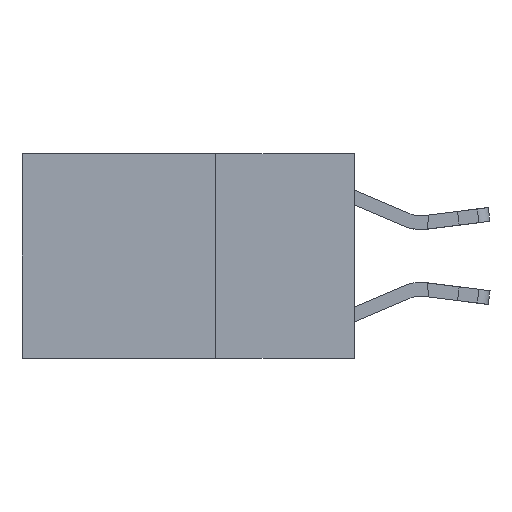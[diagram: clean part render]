
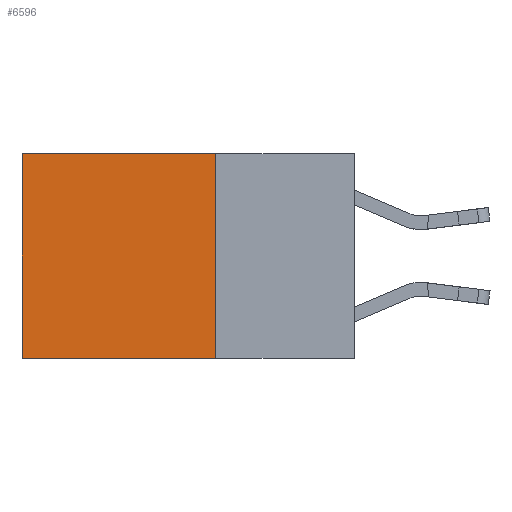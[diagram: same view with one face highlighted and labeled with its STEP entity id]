
A CAD part, left-side view. The second image highlights one B-rep face of the part: STEP entity #6596.
In plain terms, the highlighted planar face has unit normal (-1, 0, 0).
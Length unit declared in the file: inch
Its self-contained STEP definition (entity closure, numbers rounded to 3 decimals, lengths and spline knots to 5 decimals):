
#45 = FACE_OUTER_BOUND ( 'NONE', #14893, .T. ) ;
#304 = ORIENTED_EDGE ( 'NONE', *, *, #19773, .T. ) ;
#1664 = EDGE_CURVE ( 'NONE', #19805, #15341, #19872, .T. ) ;
#1724 = CARTESIAN_POINT ( 'NONE',  ( 0.2625, 0.25, 0. ) ) ;
#1777 = CARTESIAN_POINT ( 'NONE',  ( 0.2625, 0.25, -0.37 ) ) ;
#2190 = VECTOR ( 'NONE', #11734, 39.37008 ) ;
#2728 = LINE ( 'NONE', #18237, #15926 ) ;
#4060 = CARTESIAN_POINT ( 'NONE',  ( 0.2625, 0.6, -0.37 ) ) ;
#5270 = CARTESIAN_POINT ( 'NONE',  ( 0.2625, 0.25, -0.37 ) ) ;
#6333 = ORIENTED_EDGE ( 'NONE', *, *, #1664, .F. ) ;
#6501 = DIRECTION ( 'NONE',  ( 1., 0., 0. ) ) ;
#6596 = ADVANCED_FACE ( 'NONE', ( #45 ), #16351, .F. ) ;
#8082 = CARTESIAN_POINT ( 'NONE',  ( 0.2625, 0.25, 0. ) ) ;
#8401 = DIRECTION ( 'NONE',  ( 0., 0., -1. ) ) ;
#9486 = CARTESIAN_POINT ( 'NONE',  ( 0.2625, 0.6, 0. ) ) ;
#9937 = VERTEX_POINT ( 'NONE', #9486 ) ;
#11339 = ORIENTED_EDGE ( 'NONE', *, *, #17902, .T. ) ;
#11662 = CARTESIAN_POINT ( 'NONE',  ( 0.2625, 0.6, 0. ) ) ;
#11734 = DIRECTION ( 'NONE',  ( 0., 0., -1. ) ) ;
#13450 = CARTESIAN_POINT ( 'NONE',  ( 0.2625, 0.25, 0. ) ) ;
#13697 = VECTOR ( 'NONE', #20006, 39.37008 ) ;
#14215 = LINE ( 'NONE', #13450, #13697 ) ;
#14893 = EDGE_LOOP ( 'NONE', ( #11339, #6333, #18866, #304 ) ) ;
#15051 = VECTOR ( 'NONE', #18351, 39.37008 ) ;
#15341 = VERTEX_POINT ( 'NONE', #4060 ) ;
#15675 = VERTEX_POINT ( 'NONE', #1724 ) ;
#15926 = VECTOR ( 'NONE', #8401, 39.37008 ) ;
#16351 = PLANE ( 'NONE',  #20102 ) ;
#17899 = EDGE_CURVE ( 'NONE', #15675, #19805, #2728, .T. ) ;
#17902 = EDGE_CURVE ( 'NONE', #9937, #15341, #19756, .T. ) ;
#17992 = DIRECTION ( 'NONE',  ( 0., 0., -1. ) ) ;
#18237 = CARTESIAN_POINT ( 'NONE',  ( 0.2625, 0.25, 0. ) ) ;
#18351 = DIRECTION ( 'NONE',  ( 0., 1., 0. ) ) ;
#18866 = ORIENTED_EDGE ( 'NONE', *, *, #17899, .F. ) ;
#19756 = LINE ( 'NONE', #11662, #2190 ) ;
#19773 = EDGE_CURVE ( 'NONE', #15675, #9937, #14215, .T. ) ;
#19805 = VERTEX_POINT ( 'NONE', #5270 ) ;
#19872 = LINE ( 'NONE', #1777, #15051 ) ;
#20006 = DIRECTION ( 'NONE',  ( 0., 1., 0. ) ) ;
#20102 = AXIS2_PLACEMENT_3D ( 'NONE', #8082, #6501, #17992 ) ;
